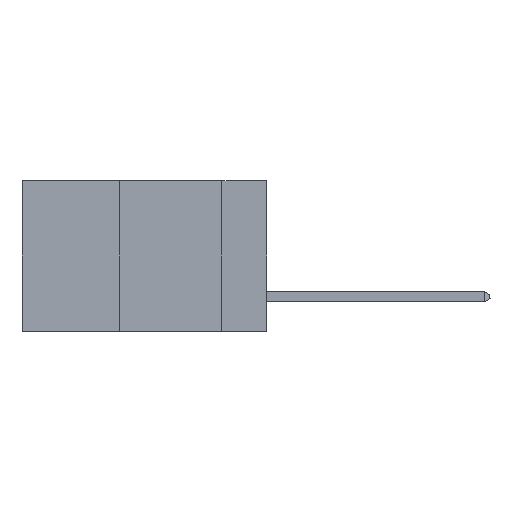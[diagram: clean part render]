
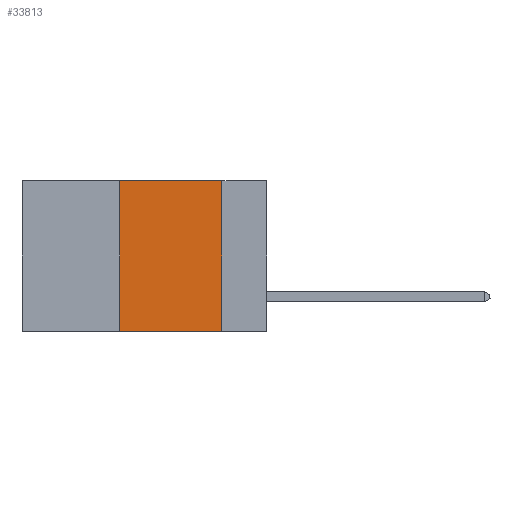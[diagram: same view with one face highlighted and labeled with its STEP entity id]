
A CAD part, left-side view. The second image highlights one B-rep face of the part: STEP entity #33813.
In plain terms, the highlighted planar face has unit normal (-1, 0, 0).
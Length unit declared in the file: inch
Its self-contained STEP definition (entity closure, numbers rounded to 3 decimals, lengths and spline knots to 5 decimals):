
#420 = ORIENTED_EDGE ( 'NONE', *, *, #14511, .F. ) ;
#486 = LINE ( 'NONE', #23348, #28863 ) ;
#3419 = VECTOR ( 'NONE', #6040, 39.37008 ) ;
#3724 = DIRECTION ( 'NONE',  ( 0., -1., 0. ) ) ;
#4083 = LINE ( 'NONE', #18724, #18310 ) ;
#4301 = LINE ( 'NONE', #31598, #3419 ) ;
#4415 = EDGE_CURVE ( 'NONE', #5120, #32257, #4301, .T. ) ;
#5120 = VERTEX_POINT ( 'NONE', #16905 ) ;
#6040 = DIRECTION ( 'NONE',  ( 0., 0., -1. ) ) ;
#6675 = LINE ( 'NONE', #25831, #24922 ) ;
#8737 = EDGE_CURVE ( 'NONE', #31200, #25848, #4083, .T. ) ;
#12728 = ORIENTED_EDGE ( 'NONE', *, *, #8737, .F. ) ;
#13708 = CARTESIAN_POINT ( 'NONE',  ( 0., 0.36, 0. ) ) ;
#14511 = EDGE_CURVE ( 'NONE', #25848, #5120, #6675, .T. ) ;
#16755 = EDGE_CURVE ( 'NONE', #31200, #32257, #486, .T. ) ;
#16905 = CARTESIAN_POINT ( 'NONE',  ( 0., 0.11, 0. ) ) ;
#17527 = DIRECTION ( 'NONE',  ( 0., 0., -1. ) ) ;
#17889 = FACE_OUTER_BOUND ( 'NONE', #28010, .T. ) ;
#18310 = VECTOR ( 'NONE', #27176, 39.37008 ) ;
#18724 = CARTESIAN_POINT ( 'NONE',  ( 0., 0.36, 0. ) ) ;
#20024 = DIRECTION ( 'NONE',  ( 1., 0., 0. ) ) ;
#20052 = ORIENTED_EDGE ( 'NONE', *, *, #4415, .F. ) ;
#23348 = CARTESIAN_POINT ( 'NONE',  ( 0., 0.6, -0.37 ) ) ;
#24642 = CARTESIAN_POINT ( 'NONE',  ( 0., 0.36, -0.37 ) ) ;
#24922 = VECTOR ( 'NONE', #25952, 39.37008 ) ;
#25648 = CARTESIAN_POINT ( 'NONE',  ( 0., 0.6, 0. ) ) ;
#25831 = CARTESIAN_POINT ( 'NONE',  ( 0., 0.6, 0. ) ) ;
#25848 = VERTEX_POINT ( 'NONE', #13708 ) ;
#25952 = DIRECTION ( 'NONE',  ( 0., -1., 0. ) ) ;
#26156 = ORIENTED_EDGE ( 'NONE', *, *, #16755, .T. ) ;
#27176 = DIRECTION ( 'NONE',  ( 0., 0., 1. ) ) ;
#28010 = EDGE_LOOP ( 'NONE', ( #20052, #420, #12728, #26156 ) ) ;
#28863 = VECTOR ( 'NONE', #3724, 39.37008 ) ;
#30192 = AXIS2_PLACEMENT_3D ( 'NONE', #25648, #20024, #17527 ) ;
#31200 = VERTEX_POINT ( 'NONE', #24642 ) ;
#31598 = CARTESIAN_POINT ( 'NONE',  ( 0., 0.11, 0. ) ) ;
#32257 = VERTEX_POINT ( 'NONE', #35215 ) ;
#33813 = ADVANCED_FACE ( 'NONE', ( #17889 ), #34565, .F. ) ;
#34565 = PLANE ( 'NONE',  #30192 ) ;
#35215 = CARTESIAN_POINT ( 'NONE',  ( 0., 0.11, -0.37 ) ) ;
